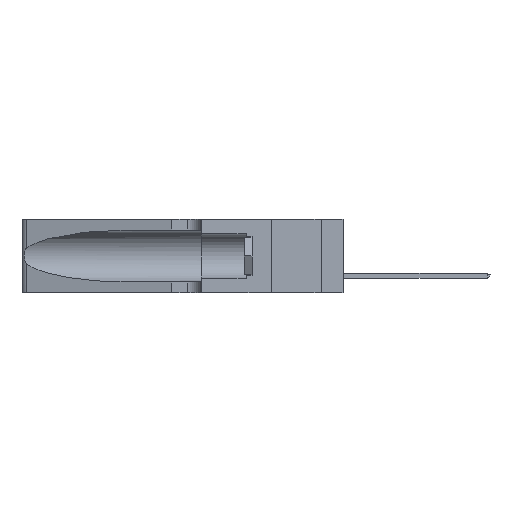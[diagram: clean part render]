
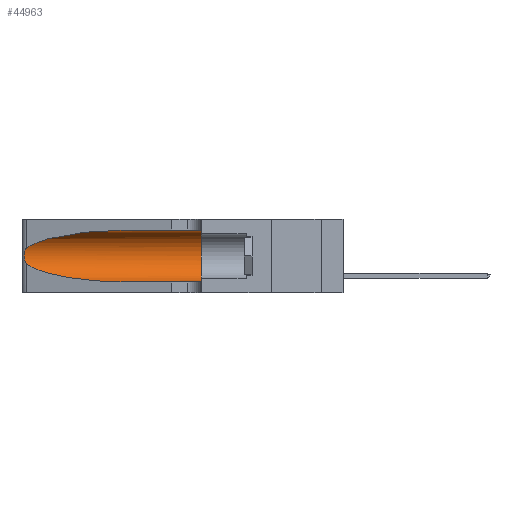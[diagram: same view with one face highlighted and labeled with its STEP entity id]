
A CAD part, left-side view. The second image highlights one B-rep face of the part: STEP entity #44963.
In plain terms, the highlighted cylindrical face has radius 3.308 mm (diameter 6.617 mm), a partial arc.
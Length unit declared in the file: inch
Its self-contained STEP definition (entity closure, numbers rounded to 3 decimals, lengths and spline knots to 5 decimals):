
#161 = ORIENTED_EDGE ( 'NONE', *, *, #19916, .T. ) ;
#497 = ORIENTED_EDGE ( 'NONE', *, *, #38540, .T. ) ;
#783 = CARTESIAN_POINT ( 'NONE',  ( 0.1305, 1.61858, 0.185 ) ) ;
#1058 = CIRCLE ( 'NONE', #7656, 0.13025 ) ;
#2518 = ORIENTED_EDGE ( 'NONE', *, *, #49129, .T. ) ;
#3721 = CARTESIAN_POINT ( 'NONE',  ( 0.2373, 1.15595, 0.08982 ) ) ;
#4120 = CARTESIAN_POINT ( 'NONE',  ( 0.25487, 1.22718, 0.22369 ) ) ;
#4394 = CARTESIAN_POINT ( 'NONE',  ( 0.1305, 0.35, 0.05475 ) ) ;
#4451 = CARTESIAN_POINT ( 'NONE',  ( 0.25787, 1.23484, 0.2124 ) ) ;
#4501 = VECTOR ( 'NONE', #40606, 39.37008 ) ;
#5195 = VERTEX_POINT ( 'NONE', #4394 ) ;
#7404 = CARTESIAN_POINT ( 'NONE',  ( 0.1305, 0.72297, 0.05475 ) ) ;
#7656 = AXIS2_PLACEMENT_3D ( 'NONE', #50719, #44043, #11426 ) ;
#8525 = CARTESIAN_POINT ( 'NONE',  ( 0.26017, 1.23833, 0.17102 ) ) ;
#10474 = LINE ( 'NONE', #50347, #52335 ) ;
#10574 = EDGE_CURVE ( 'NONE', #22604, #16730, #47564, .T. ) ;
#11426 = DIRECTION ( 'NONE',  ( 0., 0., 1. ) ) ;
#11891 = ORIENTED_EDGE ( 'NONE', *, *, #38160, .T. ) ;
#13034 = AXIS2_PLACEMENT_3D ( 'NONE', #783, #13529, #38210 ) ;
#13529 = DIRECTION ( 'NONE',  ( 0., -1., 0. ) ) ;
#16730 = VERTEX_POINT ( 'NONE', #27274 ) ;
#17059 = FACE_OUTER_BOUND ( 'NONE', #49186, .T. ) ;
#19916 = EDGE_CURVE ( 'NONE', #22604, #44203, #36896, .T. ) ;
#20521 = CARTESIAN_POINT ( 'NONE',  ( 0.25639, 1.23186, 0.15144 ) ) ;
#20838 = CARTESIAN_POINT ( 'NONE',  ( 0.26075, 1.23896, 0.19203 ) ) ;
#22604 = VERTEX_POINT ( 'NONE', #50164 ) ;
#24574 = CARTESIAN_POINT ( 'NONE',  ( 0.25487, 1.22718, 0.14631 ) ) ;
#26393 = CARTESIAN_POINT ( 'NONE',  ( 0.2373, 1.15595, 0.28018 ) ) ;
#27220 = CARTESIAN_POINT ( 'NONE',  ( 0.25639, 1.23184, 0.21858 ) ) ;
#27274 = CARTESIAN_POINT ( 'NONE',  ( 0.1305, 0.35, 0.31525 ) ) ;
#27565 = CARTESIAN_POINT ( 'NONE',  ( 0.25555, 1.22993, 0.14849 ) ) ;
#29661 = ORIENTED_EDGE ( 'NONE', *, *, #41563, .F. ) ;
#31678 = CYLINDRICAL_SURFACE ( 'NONE', #13034, 0.13025 ) ;
#31857 = CARTESIAN_POINT ( 'NONE',  ( 0.26018, 1.23835, 0.19895 ) ) ;
#31985 = CARTESIAN_POINT ( 'NONE',  ( 0.1305, 0.72297, 0.05475 ) ) ;
#34518 = CARTESIAN_POINT ( 'NONE',  ( 0.25487, 1.22718, 0.22369 ) ) ;
#35192 = CARTESIAN_POINT ( 'NONE',  ( 0.25487, 1.22718, 0.22369 ) ) ;
#36896 =( BOUNDED_CURVE ( )  B_SPLINE_CURVE ( 3, ( #43282, #50679, #26393, #34518 ),
 .UNSPECIFIED., .F., .F. ) 
 B_SPLINE_CURVE_WITH_KNOTS ( ( 4, 4 ),
 ( 1.5708, 2.84003 ),
 .UNSPECIFIED. ) 
 CURVE ( )  GEOMETRIC_REPRESENTATION_ITEM ( )  RATIONAL_B_SPLINE_CURVE ( ( 1., 0.87, 0.87, 1. ) ) 
 REPRESENTATION_ITEM ( '' )  );
#37643 = CARTESIAN_POINT ( 'NONE',  ( 0.25487, 1.22718, 0.14631 ) ) ;
#38160 = EDGE_CURVE ( 'NONE', #46308, #5195, #10474, .T. ) ;
#38210 = DIRECTION ( 'NONE',  ( 0., 0., -1. ) ) ;
#38509 = CARTESIAN_POINT ( 'NONE',  ( 0.25487, 1.22718, 0.14631 ) ) ;
#38540 = EDGE_CURVE ( 'NONE', #50640, #46308, #51962, .T. ) ;
#40134 = CARTESIAN_POINT ( 'NONE',  ( 0.1305, 1.61858, 0.31525 ) ) ;
#40606 = DIRECTION ( 'NONE',  ( 0., -1., 0. ) ) ;
#40835 = CARTESIAN_POINT ( 'NONE',  ( 0.25856, 1.23593, 0.16098 ) ) ;
#41563 = EDGE_CURVE ( 'NONE', #16730, #5195, #1058, .T. ) ;
#42573 = DIRECTION ( 'NONE',  ( 0., -1., 0. ) ) ;
#43282 = CARTESIAN_POINT ( 'NONE',  ( 0.1305, 0.72297, 0.31525 ) ) ;
#43408 = CARTESIAN_POINT ( 'NONE',  ( 0.25555, 1.22994, 0.2215 ) ) ;
#44043 = DIRECTION ( 'NONE',  ( 0., 1., 0. ) ) ;
#44134 = B_SPLINE_CURVE_WITH_KNOTS ( 'NONE', 3,
 ( #35192, #43408, #27220, #4451, #51938, #31857, #20838, #47982, #8525, #40835, #45109, #20521, #27565, #24574 ),
 .UNSPECIFIED., .F., .F.,
 ( 4, 2, 2, 2, 2, 2, 4 ),
 ( 0., 0.00027, 0.00053, 0.00107, 0.0016, 0.00187, 0.00214 ),
 .UNSPECIFIED. ) ;
#44203 = VERTEX_POINT ( 'NONE', #4120 ) ;
#44963 = ADVANCED_FACE ( 'NONE', ( #17059 ), #31678, .F. ) ;
#45109 = CARTESIAN_POINT ( 'NONE',  ( 0.25789, 1.23486, 0.15765 ) ) ;
#46308 = VERTEX_POINT ( 'NONE', #7404 ) ;
#47564 = LINE ( 'NONE', #40134, #4501 ) ;
#47982 = CARTESIAN_POINT ( 'NONE',  ( 0.26075, 1.23896, 0.178 ) ) ;
#48281 = CARTESIAN_POINT ( 'NONE',  ( 0.18966, 0.96281, 0.05475 ) ) ;
#49129 = EDGE_CURVE ( 'NONE', #44203, #50640, #44134, .T. ) ;
#49186 = EDGE_LOOP ( 'NONE', ( #161, #2518, #497, #11891, #29661, #51269 ) ) ;
#50164 = CARTESIAN_POINT ( 'NONE',  ( 0.1305, 0.72297, 0.31525 ) ) ;
#50347 = CARTESIAN_POINT ( 'NONE',  ( 0.1305, 1.61858, 0.05475 ) ) ;
#50640 = VERTEX_POINT ( 'NONE', #37643 ) ;
#50679 = CARTESIAN_POINT ( 'NONE',  ( 0.18966, 0.96281, 0.31525 ) ) ;
#50719 = CARTESIAN_POINT ( 'NONE',  ( 0.1305, 0.35, 0.185 ) ) ;
#51269 = ORIENTED_EDGE ( 'NONE', *, *, #10574, .F. ) ;
#51938 = CARTESIAN_POINT ( 'NONE',  ( 0.25854, 1.2359, 0.20912 ) ) ;
#51962 =( BOUNDED_CURVE ( )  B_SPLINE_CURVE ( 3, ( #38509, #3721, #48281, #31985 ),
 .UNSPECIFIED., .F., .F. ) 
 B_SPLINE_CURVE_WITH_KNOTS ( ( 4, 4 ),
 ( 3.44316, 4.71239 ),
 .UNSPECIFIED. ) 
 CURVE ( )  GEOMETRIC_REPRESENTATION_ITEM ( )  RATIONAL_B_SPLINE_CURVE ( ( 1., 0.87, 0.87, 1. ) ) 
 REPRESENTATION_ITEM ( '' )  );
#52335 = VECTOR ( 'NONE', #42573, 39.37008 ) ;
